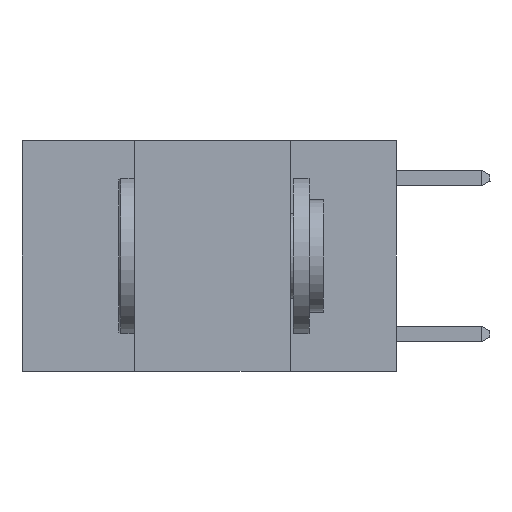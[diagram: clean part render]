
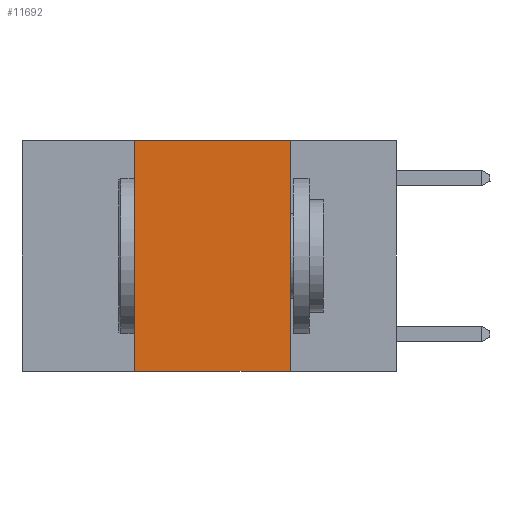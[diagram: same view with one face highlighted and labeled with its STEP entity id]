
A CAD part, left-side view. The second image highlights one B-rep face of the part: STEP entity #11692.
In plain terms, the highlighted planar face has unit normal (-1, 0, 0).
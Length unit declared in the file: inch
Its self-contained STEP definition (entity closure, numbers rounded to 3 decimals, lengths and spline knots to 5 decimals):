
#162 = ORIENTED_EDGE ( 'NONE', *, *, #5695, .F. ) ;
#1327 = DIRECTION ( 'NONE',  ( 0., 0., -1. ) ) ;
#1813 = AXIS2_PLACEMENT_3D ( 'NONE', #12566, #13859, #6193 ) ;
#1849 = CARTESIAN_POINT ( 'NONE',  ( 0., 0.42, 0. ) ) ;
#3390 = LINE ( 'NONE', #7894, #6443 ) ;
#3439 = VERTEX_POINT ( 'NONE', #9324 ) ;
#3570 = PLANE ( 'NONE',  #1813 ) ;
#3682 = VERTEX_POINT ( 'NONE', #1849 ) ;
#4180 = ORIENTED_EDGE ( 'NONE', *, *, #5049, .T. ) ;
#4789 = ORIENTED_EDGE ( 'NONE', *, *, #10940, .F. ) ;
#5049 = EDGE_CURVE ( 'NONE', #13411, #3439, #5086, .T. ) ;
#5086 = LINE ( 'NONE', #8143, #11454 ) ;
#5463 = LINE ( 'NONE', #6156, #15193 ) ;
#5695 = EDGE_CURVE ( 'NONE', #5721, #3439, #3390, .T. ) ;
#5721 = VERTEX_POINT ( 'NONE', #6673 ) ;
#6156 = CARTESIAN_POINT ( 'NONE',  ( 0., 0.6, 0. ) ) ;
#6193 = DIRECTION ( 'NONE',  ( 0., 0., -1. ) ) ;
#6216 = DIRECTION ( 'NONE',  ( 0., -1., 0. ) ) ;
#6425 = FACE_OUTER_BOUND ( 'NONE', #13128, .T. ) ;
#6443 = VECTOR ( 'NONE', #1327, 39.37008 ) ;
#6673 = CARTESIAN_POINT ( 'NONE',  ( 0., 0.17, 0. ) ) ;
#7894 = CARTESIAN_POINT ( 'NONE',  ( 0., 0.17, 0. ) ) ;
#8143 = CARTESIAN_POINT ( 'NONE',  ( 0., 0.6, -0.37 ) ) ;
#8425 = EDGE_CURVE ( 'NONE', #13411, #3682, #12609, .T. ) ;
#9173 = VECTOR ( 'NONE', #14386, 39.37008 ) ;
#9324 = CARTESIAN_POINT ( 'NONE',  ( 0., 0.17, -0.37 ) ) ;
#9403 = DIRECTION ( 'NONE',  ( 0., -1., 0. ) ) ;
#10940 = EDGE_CURVE ( 'NONE', #3682, #5721, #5463, .T. ) ;
#11454 = VECTOR ( 'NONE', #9403, 39.37008 ) ;
#11692 = ADVANCED_FACE ( 'NONE', ( #6425 ), #3570, .F. ) ;
#12566 = CARTESIAN_POINT ( 'NONE',  ( 0., 0.6, 0. ) ) ;
#12609 = LINE ( 'NONE', #16814, #9173 ) ;
#13128 = EDGE_LOOP ( 'NONE', ( #162, #4789, #13303, #4180 ) ) ;
#13303 = ORIENTED_EDGE ( 'NONE', *, *, #8425, .F. ) ;
#13411 = VERTEX_POINT ( 'NONE', #16679 ) ;
#13859 = DIRECTION ( 'NONE',  ( 1., 0., 0. ) ) ;
#14386 = DIRECTION ( 'NONE',  ( 0., 0., 1. ) ) ;
#15193 = VECTOR ( 'NONE', #6216, 39.37008 ) ;
#16679 = CARTESIAN_POINT ( 'NONE',  ( 0., 0.42, -0.37 ) ) ;
#16814 = CARTESIAN_POINT ( 'NONE',  ( 0., 0.42, 0. ) ) ;
